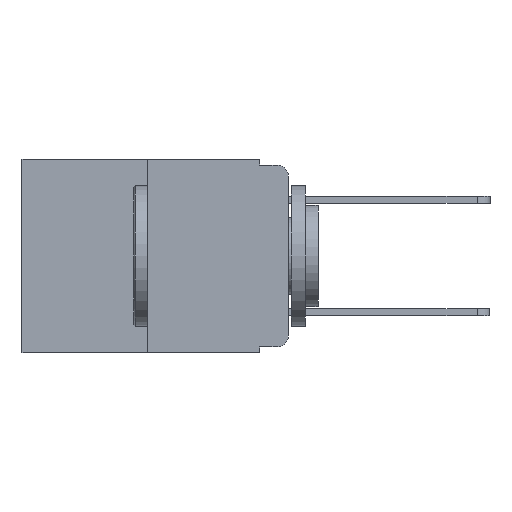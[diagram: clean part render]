
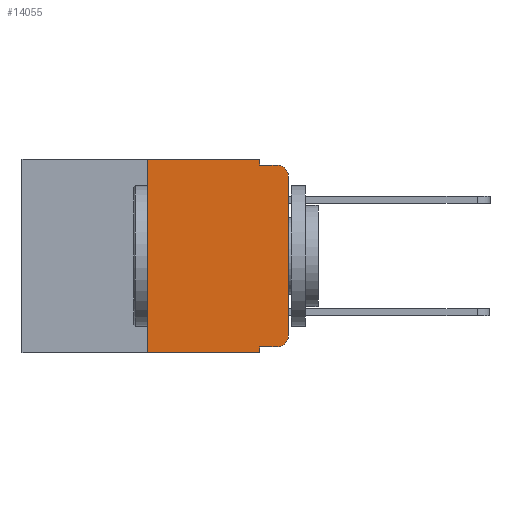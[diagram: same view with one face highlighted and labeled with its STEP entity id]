
A CAD part, left-side view. The second image highlights one B-rep face of the part: STEP entity #14055.
In plain terms, the highlighted planar face has unit normal (-1, 0, 0).
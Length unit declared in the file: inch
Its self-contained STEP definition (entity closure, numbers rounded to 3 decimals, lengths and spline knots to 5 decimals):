
#174 = VERTEX_POINT ( 'NONE', #12526 ) ;
#405 = CARTESIAN_POINT ( 'NONE',  ( 0., 0.051, -0.343 ) ) ;
#612 = DIRECTION ( 'NONE',  ( 0., 0., -1. ) ) ;
#1046 = VERTEX_POINT ( 'NONE', #19512 ) ;
#1053 = VERTEX_POINT ( 'NONE', #8287 ) ;
#1223 = EDGE_CURVE ( 'NONE', #174, #17819, #3491, .T. ) ;
#1230 = AXIS2_PLACEMENT_3D ( 'NONE', #4100, #15919, #5878 ) ;
#1993 = CARTESIAN_POINT ( 'NONE',  ( 0., 0.051, -0.01 ) ) ;
#2202 = AXIS2_PLACEMENT_3D ( 'NONE', #5929, #10083, #5898 ) ;
#2327 = VERTEX_POINT ( 'NONE', #20317 ) ;
#2883 = LINE ( 'NONE', #17695, #20031 ) ;
#2936 = CARTESIAN_POINT ( 'NONE',  ( 0., 0., 0. ) ) ;
#3165 = VECTOR ( 'NONE', #17037, 39.37008 ) ;
#3491 = LINE ( 'NONE', #4884, #17901 ) ;
#3915 = EDGE_CURVE ( 'NONE', #2327, #8293, #21068, .T. ) ;
#4100 = CARTESIAN_POINT ( 'NONE',  ( 0., 0.02, -0.03 ) ) ;
#4205 = CARTESIAN_POINT ( 'NONE',  ( 0., 0.051, 0. ) ) ;
#4810 = CARTESIAN_POINT ( 'NONE',  ( 0., 0.051, -0.01 ) ) ;
#4884 = CARTESIAN_POINT ( 'NONE',  ( 0., 0.473, -0.343 ) ) ;
#5033 = VERTEX_POINT ( 'NONE', #15364 ) ;
#5093 = EDGE_CURVE ( 'NONE', #1046, #2327, #7944, .T. ) ;
#5803 = ORIENTED_EDGE ( 'NONE', *, *, #14226, .F. ) ;
#5878 = DIRECTION ( 'NONE',  ( 0., 0., -1. ) ) ;
#5898 = DIRECTION ( 'NONE',  ( 0., 0., -1. ) ) ;
#5929 = CARTESIAN_POINT ( 'NONE',  ( 0., 0.02, -0.313 ) ) ;
#6133 = DIRECTION ( 'NONE',  ( 0., 0., 1. ) ) ;
#6302 = CARTESIAN_POINT ( 'NONE',  ( 0., 0.25, 0. ) ) ;
#6478 = ORIENTED_EDGE ( 'NONE', *, *, #11027, .F. ) ;
#6714 = VERTEX_POINT ( 'NONE', #8344 ) ;
#6988 = VERTEX_POINT ( 'NONE', #1993 ) ;
#7156 = CARTESIAN_POINT ( 'NONE',  ( 0., 0.473, 0. ) ) ;
#7183 = CARTESIAN_POINT ( 'NONE',  ( 0., 0.051, -0.333 ) ) ;
#7258 = ORIENTED_EDGE ( 'NONE', *, *, #15075, .F. ) ;
#7584 = LINE ( 'NONE', #13125, #12147 ) ;
#7944 = LINE ( 'NONE', #7183, #3165 ) ;
#8010 = VECTOR ( 'NONE', #8944, 39.37008 ) ;
#8287 = CARTESIAN_POINT ( 'NONE',  ( 0., 0., -0.03 ) ) ;
#8293 = VERTEX_POINT ( 'NONE', #11574 ) ;
#8344 = CARTESIAN_POINT ( 'NONE',  ( 0., 0.051, 0. ) ) ;
#8529 = ORIENTED_EDGE ( 'NONE', *, *, #9884, .F. ) ;
#8691 = EDGE_CURVE ( 'NONE', #1046, #17819, #9405, .T. ) ;
#8720 = ORIENTED_EDGE ( 'NONE', *, *, #1223, .T. ) ;
#8794 = DIRECTION ( 'NONE',  ( 0., -1., 0. ) ) ;
#8944 = DIRECTION ( 'NONE',  ( 0., -1., 0. ) ) ;
#9293 = ORIENTED_EDGE ( 'NONE', *, *, #16336, .T. ) ;
#9405 = LINE ( 'NONE', #4205, #17450 ) ;
#9884 = EDGE_CURVE ( 'NONE', #174, #12838, #2883, .T. ) ;
#10083 = DIRECTION ( 'NONE',  ( -1., 0., 0. ) ) ;
#10120 = DIRECTION ( 'NONE',  ( 0., -1., 0. ) ) ;
#10996 = VECTOR ( 'NONE', #16487, 39.37008 ) ;
#11027 = EDGE_CURVE ( 'NONE', #6714, #6988, #7584, .T. ) ;
#11212 = ORIENTED_EDGE ( 'NONE', *, *, #15323, .T. ) ;
#11424 = DIRECTION ( 'NONE',  ( 1., 0., 0. ) ) ;
#11574 = CARTESIAN_POINT ( 'NONE',  ( 0., 0., -0.313 ) ) ;
#11670 = ORIENTED_EDGE ( 'NONE', *, *, #8691, .F. ) ;
#12147 = VECTOR ( 'NONE', #17803, 39.37008 ) ;
#12524 = LINE ( 'NONE', #7156, #8010 ) ;
#12526 = CARTESIAN_POINT ( 'NONE',  ( 0., 0.25, -0.343 ) ) ;
#12824 = DIRECTION ( 'NONE',  ( 0., 0., -1. ) ) ;
#12838 = VERTEX_POINT ( 'NONE', #6302 ) ;
#13125 = CARTESIAN_POINT ( 'NONE',  ( 0., 0.051, 0. ) ) ;
#13542 = FACE_OUTER_BOUND ( 'NONE', #20722, .T. ) ;
#14055 = ADVANCED_FACE ( 'NONE', ( #13542 ), #17712, .F. ) ;
#14226 = EDGE_CURVE ( 'NONE', #6988, #5033, #15318, .T. ) ;
#14616 = ORIENTED_EDGE ( 'NONE', *, *, #5093, .T. ) ;
#14914 = ORIENTED_EDGE ( 'NONE', *, *, #3915, .T. ) ;
#15075 = EDGE_CURVE ( 'NONE', #12838, #6714, #12524, .T. ) ;
#15318 = LINE ( 'NONE', #4810, #18919 ) ;
#15323 = EDGE_CURVE ( 'NONE', #1053, #5033, #17922, .T. ) ;
#15364 = CARTESIAN_POINT ( 'NONE',  ( 0., 0.02, -0.01 ) ) ;
#15919 = DIRECTION ( 'NONE',  ( -1., 0., 0. ) ) ;
#16158 = CARTESIAN_POINT ( 'NONE',  ( 0., 0.473, 0. ) ) ;
#16336 = EDGE_CURVE ( 'NONE', #8293, #1053, #20305, .T. ) ;
#16487 = DIRECTION ( 'NONE',  ( 0., 0., 1. ) ) ;
#17037 = DIRECTION ( 'NONE',  ( 0., -1., 0. ) ) ;
#17450 = VECTOR ( 'NONE', #12824, 39.37008 ) ;
#17695 = CARTESIAN_POINT ( 'NONE',  ( 0., 0.25, 0. ) ) ;
#17712 = PLANE ( 'NONE',  #20478 ) ;
#17803 = DIRECTION ( 'NONE',  ( 0., 0., -1. ) ) ;
#17819 = VERTEX_POINT ( 'NONE', #405 ) ;
#17901 = VECTOR ( 'NONE', #8794, 39.37008 ) ;
#17922 = CIRCLE ( 'NONE', #1230, 0.02 ) ;
#18919 = VECTOR ( 'NONE', #10120, 39.37008 ) ;
#19512 = CARTESIAN_POINT ( 'NONE',  ( 0., 0.051, -0.333 ) ) ;
#20031 = VECTOR ( 'NONE', #6133, 39.37008 ) ;
#20305 = LINE ( 'NONE', #2936, #10996 ) ;
#20317 = CARTESIAN_POINT ( 'NONE',  ( 0., 0.02, -0.333 ) ) ;
#20478 = AXIS2_PLACEMENT_3D ( 'NONE', #16158, #11424, #612 ) ;
#20722 = EDGE_LOOP ( 'NONE', ( #9293, #11212, #5803, #6478, #7258, #8529, #8720, #11670, #14616, #14914 ) ) ;
#21068 = CIRCLE ( 'NONE', #2202, 0.02 ) ;
